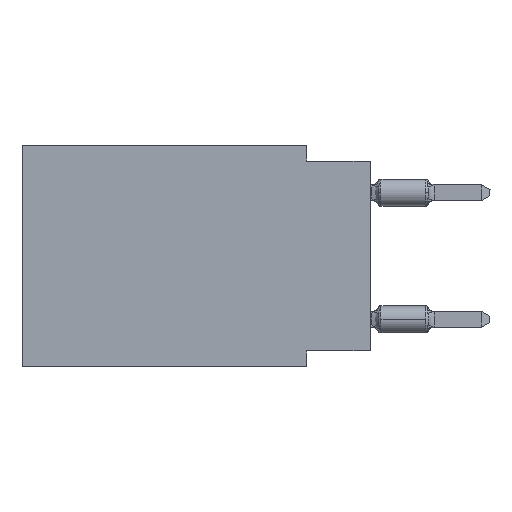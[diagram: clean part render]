
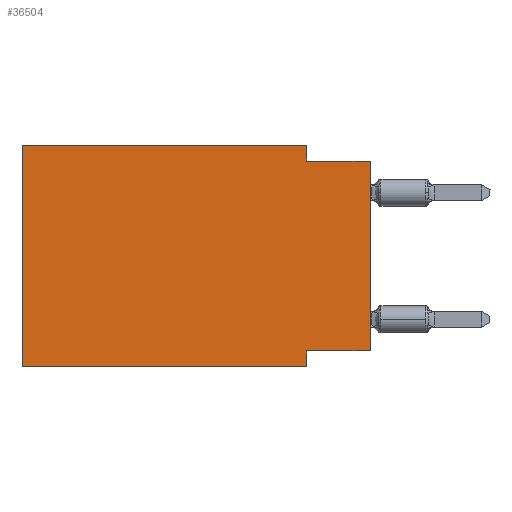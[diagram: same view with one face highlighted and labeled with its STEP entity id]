
A CAD part, left-side view. The second image highlights one B-rep face of the part: STEP entity #36504.
In plain terms, the highlighted planar face has unit normal (-1, 0, 0).
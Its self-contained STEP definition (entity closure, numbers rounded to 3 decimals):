
#1083 = LINE ( 'NONE', #15063, #25229 ) ;
#1303 = VERTEX_POINT ( 'NONE', #5535 ) ;
#1699 = DIRECTION ( 'NONE',  ( 0., 0., -1. ) ) ;
#1818 = ORIENTED_EDGE ( 'NONE', *, *, #51279, .F. ) ;
#4290 = LINE ( 'NONE', #18275, #28418 ) ;
#5535 = CARTESIAN_POINT ( 'NONE',  ( 0., 13.97, -8.89 ) ) ;
#5866 = AXIS2_PLACEMENT_3D ( 'NONE', #22780, #60893, #8504 ) ;
#5939 = CARTESIAN_POINT ( 'NONE',  ( 0., 2.54, -8.89 ) ) ;
#7251 = ORIENTED_EDGE ( 'NONE', *, *, #27339, .F. ) ;
#7476 = LINE ( 'NONE', #60183, #54126 ) ;
#8127 = CARTESIAN_POINT ( 'NONE',  ( 0., 0., -8.255 ) ) ;
#8504 = DIRECTION ( 'NONE',  ( 0., 0., -1. ) ) ;
#8836 = ORIENTED_EDGE ( 'NONE', *, *, #21204, .F. ) ;
#9922 = EDGE_CURVE ( 'NONE', #30637, #20692, #17151, .T. ) ;
#11382 = CARTESIAN_POINT ( 'NONE',  ( 0., 0., -0.635 ) ) ;
#13372 = CARTESIAN_POINT ( 'NONE',  ( 0., 2.54, -8.255 ) ) ;
#14961 = LINE ( 'NONE', #5939, #51504 ) ;
#15063 = CARTESIAN_POINT ( 'NONE',  ( 0., 2.54, 0. ) ) ;
#15727 = EDGE_CURVE ( 'NONE', #50497, #28529, #40202, .T. ) ;
#17151 = LINE ( 'NONE', #8127, #38851 ) ;
#18175 = CARTESIAN_POINT ( 'NONE',  ( 0., 13.97, 0. ) ) ;
#18275 = CARTESIAN_POINT ( 'NONE',  ( 0., 13.97, 0. ) ) ;
#18596 = DIRECTION ( 'NONE',  ( 0., -1., 0. ) ) ;
#18715 = VERTEX_POINT ( 'NONE', #55320 ) ;
#19297 = EDGE_LOOP ( 'NONE', ( #29629, #59663, #1818, #46433, #8836, #56342, #7251, #54047 ) ) ;
#20692 = VERTEX_POINT ( 'NONE', #13372 ) ;
#21204 = EDGE_CURVE ( 'NONE', #1303, #18715, #4290, .T. ) ;
#21350 = EDGE_CURVE ( 'NONE', #30637, #28529, #7476, .T. ) ;
#22485 = CARTESIAN_POINT ( 'NONE',  ( 0., 2.54, -8.89 ) ) ;
#22780 = CARTESIAN_POINT ( 'NONE',  ( 0., 13.97, 0. ) ) ;
#25229 = VECTOR ( 'NONE', #1699, 1000. ) ;
#26576 = DIRECTION ( 'NONE',  ( 0., -1., 0. ) ) ;
#26705 = DIRECTION ( 'NONE',  ( 0., 0., 1. ) ) ;
#27339 = EDGE_CURVE ( 'NONE', #20692, #31183, #14961, .T. ) ;
#28028 = PLANE ( 'NONE',  #5866 ) ;
#28418 = VECTOR ( 'NONE', #47368, 1000. ) ;
#28529 = VERTEX_POINT ( 'NONE', #36449 ) ;
#29629 = ORIENTED_EDGE ( 'NONE', *, *, #21350, .T. ) ;
#30637 = VERTEX_POINT ( 'NONE', #42359 ) ;
#30665 = VECTOR ( 'NONE', #42620, 1000. ) ;
#31183 = VERTEX_POINT ( 'NONE', #22485 ) ;
#34465 = DIRECTION ( 'NONE',  ( 0., 0., -1. ) ) ;
#36449 = CARTESIAN_POINT ( 'NONE',  ( 0., 0., -0.635 ) ) ;
#36504 = ADVANCED_FACE ( 'NONE', ( #50979 ), #28028, .F. ) ;
#37907 = VECTOR ( 'NONE', #26576, 1000. ) ;
#38851 = VECTOR ( 'NONE', #60513, 1000. ) ;
#40202 = LINE ( 'NONE', #11382, #37907 ) ;
#42359 = CARTESIAN_POINT ( 'NONE',  ( 0., 0., -8.255 ) ) ;
#42620 = DIRECTION ( 'NONE',  ( 0., -1., 0. ) ) ;
#44918 = VECTOR ( 'NONE', #18596, 1000. ) ;
#46433 = ORIENTED_EDGE ( 'NONE', *, *, #53218, .F. ) ;
#47249 = VERTEX_POINT ( 'NONE', #48446 ) ;
#47368 = DIRECTION ( 'NONE',  ( 0., 0., 1. ) ) ;
#48013 = EDGE_CURVE ( 'NONE', #1303, #31183, #60146, .T. ) ;
#48446 = CARTESIAN_POINT ( 'NONE',  ( 0., 2.54, 0. ) ) ;
#50497 = VERTEX_POINT ( 'NONE', #57135 ) ;
#50979 = FACE_OUTER_BOUND ( 'NONE', #19297, .T. ) ;
#51279 = EDGE_CURVE ( 'NONE', #47249, #50497, #1083, .T. ) ;
#51504 = VECTOR ( 'NONE', #34465, 1000. ) ;
#53218 = EDGE_CURVE ( 'NONE', #18715, #47249, #60637, .T. ) ;
#54047 = ORIENTED_EDGE ( 'NONE', *, *, #9922, .F. ) ;
#54126 = VECTOR ( 'NONE', #26705, 1000. ) ;
#55320 = CARTESIAN_POINT ( 'NONE',  ( 0., 13.97, 0. ) ) ;
#56342 = ORIENTED_EDGE ( 'NONE', *, *, #48013, .T. ) ;
#57135 = CARTESIAN_POINT ( 'NONE',  ( 0., 2.54, -0.635 ) ) ;
#59663 = ORIENTED_EDGE ( 'NONE', *, *, #15727, .F. ) ;
#60146 = LINE ( 'NONE', #60758, #44918 ) ;
#60183 = CARTESIAN_POINT ( 'NONE',  ( 0., 0., 0. ) ) ;
#60513 = DIRECTION ( 'NONE',  ( 0., 1., 0. ) ) ;
#60637 = LINE ( 'NONE', #18175, #30665 ) ;
#60758 = CARTESIAN_POINT ( 'NONE',  ( 0., 13.97, -8.89 ) ) ;
#60893 = DIRECTION ( 'NONE',  ( 1., 0., 0. ) ) ;
